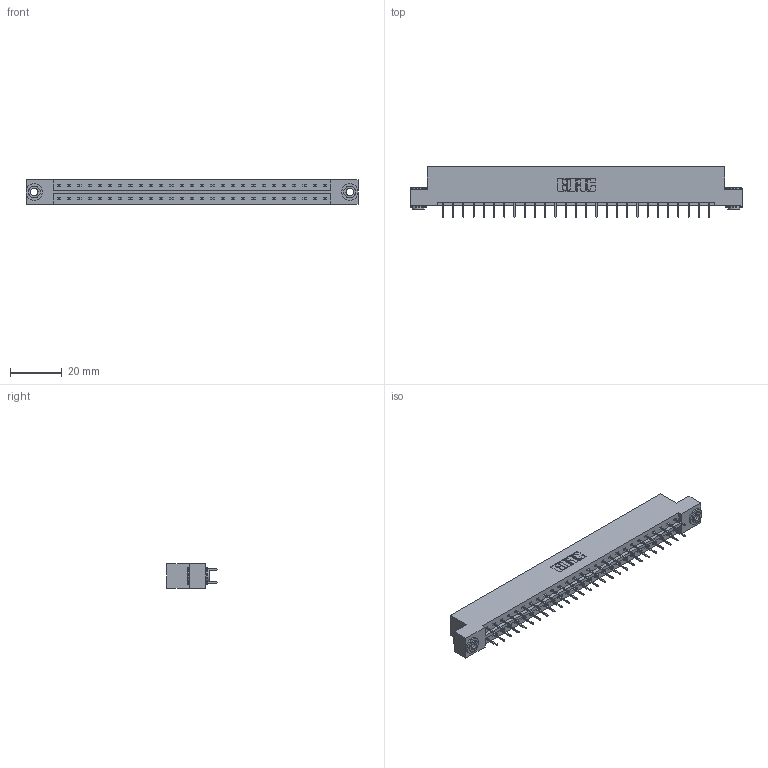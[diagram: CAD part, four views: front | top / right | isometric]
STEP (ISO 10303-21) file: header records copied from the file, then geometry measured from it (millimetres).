
FILE_DESCRIPTION (( 'STEP AP203' ), '1' );
FILE_NAME ('833-054-524-203.STEP', '2020-06-04T20:44:48', ( '' ), ( '' ), 'SwSTEP 2.0', 'SolidWorks 2020', '' );
FILE_SCHEMA (( 'CONFIG_CONTROL_DESIGN' ));
Length unit declared in the file: inch
Products named in the file (4): 345-292-001_345-293-124; 833 Part_Flush - .156 Dia - TH; 345-250-002_345-250-002-102; 833-054-524-203
Assembly tree (57 placements, depth 2):
  833-054-524-203
    833 Part_Flush - .156 Dia - TH
    345-292-001_345-293-124  x54
    345-250-002_345-250-002-102  x2
Bounding box: 128.52 x 19.69 x 9.4 mm (x, y, z)
Volume: 12919 mm3; surface area: 15087.9 mm2
Topology: 57 solids, 57 shells, 3176 faces, 8973 edges, 5762 vertices
Faces by surface type: plane 2348, cylinder 820, cone 8
Entity records: 20034 total; most frequent: CARTESIAN_POINT 3313, ORIENTED_EDGE 3242, DIRECTION 2891, EDGE_CURVE 1621, VECTOR 1473, LINE 1473, VERTEX_POINT 1074, AXIS2_PLACEMENT_3D 709
